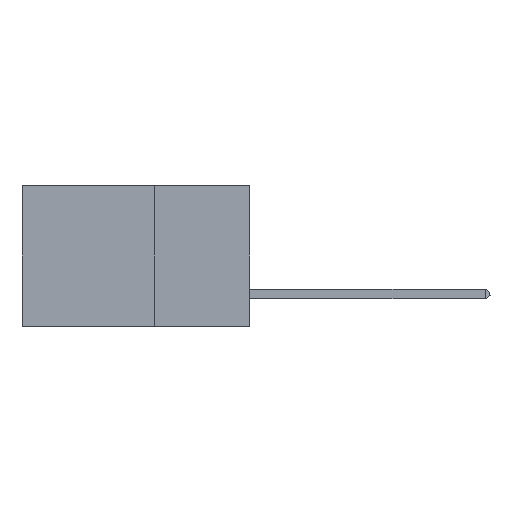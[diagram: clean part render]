
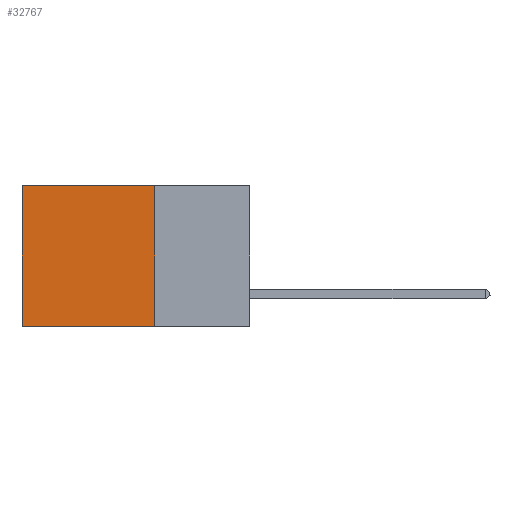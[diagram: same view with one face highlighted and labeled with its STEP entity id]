
A CAD part, left-side view. The second image highlights one B-rep face of the part: STEP entity #32767.
In plain terms, the highlighted planar face has unit normal (-1, 0, 0).
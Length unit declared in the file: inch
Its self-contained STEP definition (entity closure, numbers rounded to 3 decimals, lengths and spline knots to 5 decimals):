
#300 = CARTESIAN_POINT ( 'NONE',  ( 0.2875, 0.6, 0. ) ) ;
#4024 = DIRECTION ( 'NONE',  ( 0., 1., 0. ) ) ;
#5059 = DIRECTION ( 'NONE',  ( 0., 1., 0. ) ) ;
#5982 = VERTEX_POINT ( 'NONE', #22334 ) ;
#6922 = LINE ( 'NONE', #18708, #27180 ) ;
#7268 = EDGE_CURVE ( 'NONE', #19848, #32095, #6922, .T. ) ;
#8035 = CARTESIAN_POINT ( 'NONE',  ( 0.2875, 0.25, 0. ) ) ;
#9022 = DIRECTION ( 'NONE',  ( 0., 0., -1. ) ) ;
#11239 = CARTESIAN_POINT ( 'NONE',  ( 0.2875, 0.25, 0. ) ) ;
#11363 = LINE ( 'NONE', #34960, #34293 ) ;
#13084 = EDGE_CURVE ( 'NONE', #5982, #32095, #15003, .T. ) ;
#13362 = CARTESIAN_POINT ( 'NONE',  ( 0.2875, 0.6, -0.37 ) ) ;
#14025 = EDGE_LOOP ( 'NONE', ( #30340, #22790, #30740, #30118 ) ) ;
#14062 = DIRECTION ( 'NONE',  ( 0., 0., -1. ) ) ;
#15003 = LINE ( 'NONE', #300, #36803 ) ;
#18708 = CARTESIAN_POINT ( 'NONE',  ( 0.2875, 0.25, -0.37 ) ) ;
#19848 = VERTEX_POINT ( 'NONE', #34497 ) ;
#22334 = CARTESIAN_POINT ( 'NONE',  ( 0.2875, 0.6, 0. ) ) ;
#22441 = EDGE_CURVE ( 'NONE', #26404, #5982, #28844, .T. ) ;
#22790 = ORIENTED_EDGE ( 'NONE', *, *, #7268, .F. ) ;
#24081 = VECTOR ( 'NONE', #5059, 39.37008 ) ;
#24492 = CARTESIAN_POINT ( 'NONE',  ( 0.2875, 0.25, 0. ) ) ;
#26404 = VERTEX_POINT ( 'NONE', #8035 ) ;
#27180 = VECTOR ( 'NONE', #4024, 39.37008 ) ;
#28844 = LINE ( 'NONE', #11239, #24081 ) ;
#30105 = PLANE ( 'NONE',  #31767 ) ;
#30118 = ORIENTED_EDGE ( 'NONE', *, *, #22441, .T. ) ;
#30340 = ORIENTED_EDGE ( 'NONE', *, *, #13084, .T. ) ;
#30740 = ORIENTED_EDGE ( 'NONE', *, *, #37255, .F. ) ;
#31767 = AXIS2_PLACEMENT_3D ( 'NONE', #24492, #35718, #9022 ) ;
#32095 = VERTEX_POINT ( 'NONE', #13362 ) ;
#32441 = FACE_OUTER_BOUND ( 'NONE', #14025, .T. ) ;
#32767 = ADVANCED_FACE ( 'NONE', ( #32441 ), #30105, .F. ) ;
#34293 = VECTOR ( 'NONE', #14062, 39.37008 ) ;
#34497 = CARTESIAN_POINT ( 'NONE',  ( 0.2875, 0.25, -0.37 ) ) ;
#34960 = CARTESIAN_POINT ( 'NONE',  ( 0.2875, 0.25, 0. ) ) ;
#35718 = DIRECTION ( 'NONE',  ( 1., 0., 0. ) ) ;
#36470 = DIRECTION ( 'NONE',  ( 0., 0., -1. ) ) ;
#36803 = VECTOR ( 'NONE', #36470, 39.37008 ) ;
#37255 = EDGE_CURVE ( 'NONE', #26404, #19848, #11363, .T. ) ;
